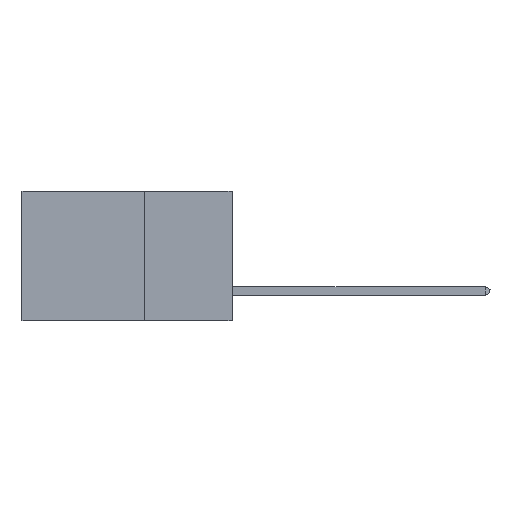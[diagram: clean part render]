
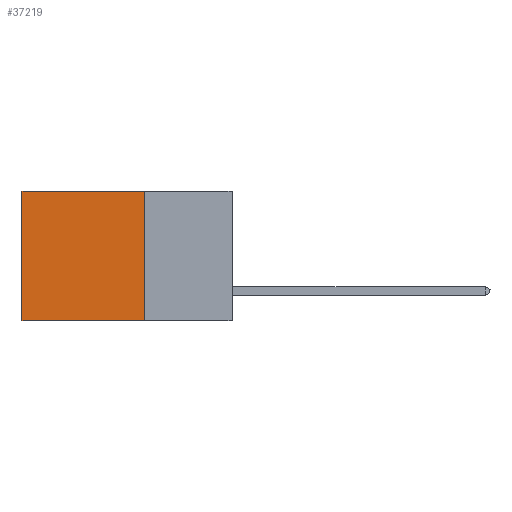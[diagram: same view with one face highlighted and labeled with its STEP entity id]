
A CAD part, left-side view. The second image highlights one B-rep face of the part: STEP entity #37219.
In plain terms, the highlighted planar face has unit normal (-1, 0, 0).
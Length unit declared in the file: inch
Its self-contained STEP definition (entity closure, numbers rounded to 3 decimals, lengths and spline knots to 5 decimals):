
#2471 = CARTESIAN_POINT ( 'NONE',  ( 0.2875, 0.6, 0. ) ) ;
#6224 = DIRECTION ( 'NONE',  ( 0., 1., 0. ) ) ;
#6313 = LINE ( 'NONE', #39502, #20300 ) ;
#6440 = CARTESIAN_POINT ( 'NONE',  ( 0.2875, 0.25, 0. ) ) ;
#6953 = DIRECTION ( 'NONE',  ( 0., 0., -1. ) ) ;
#7265 = EDGE_CURVE ( 'NONE', #13130, #18515, #11373, .T. ) ;
#9103 = CARTESIAN_POINT ( 'NONE',  ( 0.2875, 0.6, -0.37 ) ) ;
#9504 = VECTOR ( 'NONE', #6224, 39.37008 ) ;
#10603 = ORIENTED_EDGE ( 'NONE', *, *, #7265, .F. ) ;
#11373 = LINE ( 'NONE', #6440, #37970 ) ;
#11774 = CARTESIAN_POINT ( 'NONE',  ( 0.2875, 0.25, 0. ) ) ;
#12240 = ORIENTED_EDGE ( 'NONE', *, *, #27357, .F. ) ;
#12922 = AXIS2_PLACEMENT_3D ( 'NONE', #11774, #32359, #28724 ) ;
#13130 = VERTEX_POINT ( 'NONE', #48505 ) ;
#14390 = CARTESIAN_POINT ( 'NONE',  ( 0.2875, 0.25, -0.37 ) ) ;
#16861 = LINE ( 'NONE', #2471, #24585 ) ;
#16996 = CARTESIAN_POINT ( 'NONE',  ( 0.2875, 0.25, -0.37 ) ) ;
#18515 = VERTEX_POINT ( 'NONE', #14390 ) ;
#20300 = VECTOR ( 'NONE', #35758, 39.37008 ) ;
#23607 = LINE ( 'NONE', #16996, #9504 ) ;
#24585 = VECTOR ( 'NONE', #47733, 39.37008 ) ;
#26845 = PLANE ( 'NONE',  #12922 ) ;
#27357 = EDGE_CURVE ( 'NONE', #18515, #38780, #23607, .T. ) ;
#28109 = CARTESIAN_POINT ( 'NONE',  ( 0.2875, 0.6, 0. ) ) ;
#28724 = DIRECTION ( 'NONE',  ( 0., 0., -1. ) ) ;
#31555 = ORIENTED_EDGE ( 'NONE', *, *, #34704, .T. ) ;
#32359 = DIRECTION ( 'NONE',  ( 1., 0., 0. ) ) ;
#32671 = VERTEX_POINT ( 'NONE', #28109 ) ;
#34404 = ORIENTED_EDGE ( 'NONE', *, *, #43725, .T. ) ;
#34704 = EDGE_CURVE ( 'NONE', #13130, #32671, #6313, .T. ) ;
#35758 = DIRECTION ( 'NONE',  ( 0., 1., 0. ) ) ;
#37219 = ADVANCED_FACE ( 'NONE', ( #45341 ), #26845, .F. ) ;
#37970 = VECTOR ( 'NONE', #6953, 39.37008 ) ;
#38780 = VERTEX_POINT ( 'NONE', #9103 ) ;
#39502 = CARTESIAN_POINT ( 'NONE',  ( 0.2875, 0.25, 0. ) ) ;
#43725 = EDGE_CURVE ( 'NONE', #32671, #38780, #16861, .T. ) ;
#45341 = FACE_OUTER_BOUND ( 'NONE', #47516, .T. ) ;
#47516 = EDGE_LOOP ( 'NONE', ( #34404, #12240, #10603, #31555 ) ) ;
#47733 = DIRECTION ( 'NONE',  ( 0., 0., -1. ) ) ;
#48505 = CARTESIAN_POINT ( 'NONE',  ( 0.2875, 0.25, 0. ) ) ;
